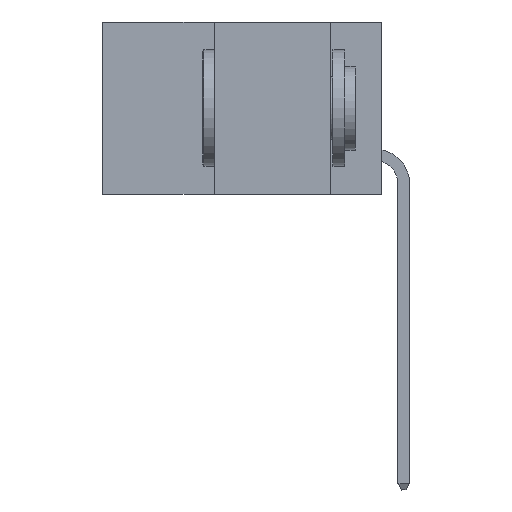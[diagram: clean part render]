
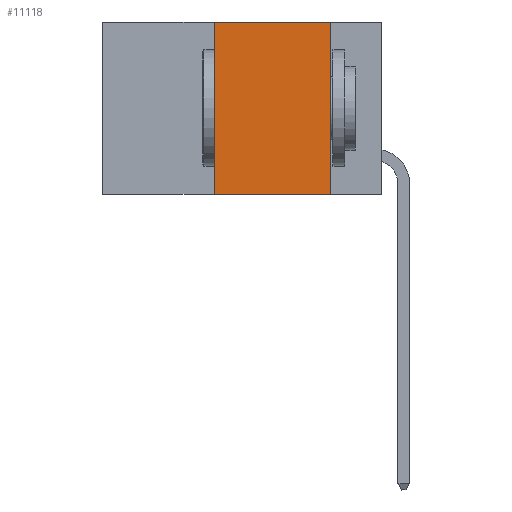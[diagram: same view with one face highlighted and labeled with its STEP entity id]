
A CAD part, left-side view. The second image highlights one B-rep face of the part: STEP entity #11118.
In plain terms, the highlighted planar face has unit normal (-1, 0, 0).
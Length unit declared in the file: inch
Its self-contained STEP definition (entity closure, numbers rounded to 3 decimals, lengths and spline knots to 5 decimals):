
#1685 = VERTEX_POINT ( 'NONE', #10008 ) ;
#1721 = DIRECTION ( 'NONE',  ( 0., -1., 0. ) ) ;
#1790 = ORIENTED_EDGE ( 'NONE', *, *, #19826, .F. ) ;
#2274 = LINE ( 'NONE', #5244, #21114 ) ;
#3397 = VERTEX_POINT ( 'NONE', #6295 ) ;
#3986 = LINE ( 'NONE', #14453, #12684 ) ;
#4019 = DIRECTION ( 'NONE',  ( 0., 0., -1. ) ) ;
#4441 = PLANE ( 'NONE',  #21320 ) ;
#4576 = LINE ( 'NONE', #5438, #15190 ) ;
#4914 = EDGE_CURVE ( 'NONE', #3397, #1685, #2274, .T. ) ;
#5244 = CARTESIAN_POINT ( 'NONE',  ( 0., 0.6, -0.37 ) ) ;
#5438 = CARTESIAN_POINT ( 'NONE',  ( 0., 0.6, 0. ) ) ;
#6067 = CARTESIAN_POINT ( 'NONE',  ( 0., 0.36, 0. ) ) ;
#6295 = CARTESIAN_POINT ( 'NONE',  ( 0., 0.36, -0.37 ) ) ;
#8444 = VECTOR ( 'NONE', #17908, 39.37008 ) ;
#10008 = CARTESIAN_POINT ( 'NONE',  ( 0., 0.11, -0.37 ) ) ;
#10055 = LINE ( 'NONE', #6067, #8444 ) ;
#10364 = VERTEX_POINT ( 'NONE', #12160 ) ;
#10464 = EDGE_CURVE ( 'NONE', #21088, #1685, #3986, .T. ) ;
#11118 = ADVANCED_FACE ( 'NONE', ( #17334 ), #4441, .F. ) ;
#11146 = CARTESIAN_POINT ( 'NONE',  ( 0., 0.6, 0. ) ) ;
#12160 = CARTESIAN_POINT ( 'NONE',  ( 0., 0.36, 0. ) ) ;
#12684 = VECTOR ( 'NONE', #4019, 39.37008 ) ;
#12711 = ORIENTED_EDGE ( 'NONE', *, *, #10464, .F. ) ;
#13728 = DIRECTION ( 'NONE',  ( 0., 0., -1. ) ) ;
#14453 = CARTESIAN_POINT ( 'NONE',  ( 0., 0.11, 0. ) ) ;
#14662 = DIRECTION ( 'NONE',  ( 0., -1., 0. ) ) ;
#14960 = EDGE_LOOP ( 'NONE', ( #12711, #1790, #20049, #18587 ) ) ;
#15190 = VECTOR ( 'NONE', #14662, 39.37008 ) ;
#17334 = FACE_OUTER_BOUND ( 'NONE', #14960, .T. ) ;
#17908 = DIRECTION ( 'NONE',  ( 0., 0., 1. ) ) ;
#18587 = ORIENTED_EDGE ( 'NONE', *, *, #4914, .T. ) ;
#18816 = DIRECTION ( 'NONE',  ( 1., 0., 0. ) ) ;
#19826 = EDGE_CURVE ( 'NONE', #10364, #21088, #4576, .T. ) ;
#20049 = ORIENTED_EDGE ( 'NONE', *, *, #22349, .F. ) ;
#21088 = VERTEX_POINT ( 'NONE', #22180 ) ;
#21114 = VECTOR ( 'NONE', #1721, 39.37008 ) ;
#21320 = AXIS2_PLACEMENT_3D ( 'NONE', #11146, #18816, #13728 ) ;
#22180 = CARTESIAN_POINT ( 'NONE',  ( 0., 0.11, 0. ) ) ;
#22349 = EDGE_CURVE ( 'NONE', #3397, #10364, #10055, .T. ) ;
